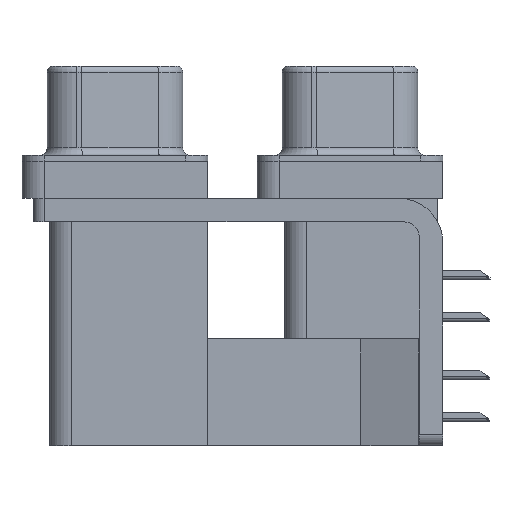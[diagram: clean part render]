
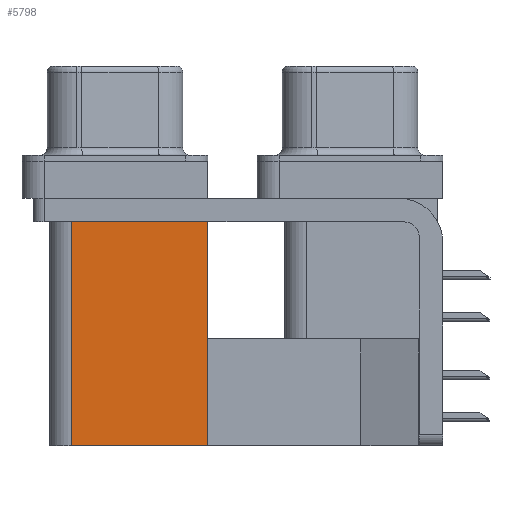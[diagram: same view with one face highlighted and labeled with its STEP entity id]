
A CAD part, left-side view. The second image highlights one B-rep face of the part: STEP entity #5798.
In plain terms, the highlighted planar face has unit normal (-1, 0, 0).
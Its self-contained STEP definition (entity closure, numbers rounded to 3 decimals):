
#100 = DIRECTION ( 'NONE',  ( 1., 0., 0. ) ) ;
#609 = VECTOR ( 'NONE', #3023, 1000. ) ;
#957 = VERTEX_POINT ( 'NONE', #12026 ) ;
#1758 = CARTESIAN_POINT ( 'NONE',  ( 3.79, 9.6, -2.5 ) ) ;
#2810 = LINE ( 'NONE', #4810, #11062 ) ;
#3023 = DIRECTION ( 'NONE',  ( 0., 0., 1. ) ) ;
#3267 = ORIENTED_EDGE ( 'NONE', *, *, #11041, .F. ) ;
#4810 = CARTESIAN_POINT ( 'NONE',  ( 3.79, 18.8, -19.2 ) ) ;
#5171 = DIRECTION ( 'NONE',  ( 0., 1., 0. ) ) ;
#5392 = FACE_OUTER_BOUND ( 'NONE', #19019, .T. ) ;
#5403 = LINE ( 'NONE', #1758, #5768 ) ;
#5515 = DIRECTION ( 'NONE',  ( 0., 0., -1. ) ) ;
#5654 = LINE ( 'NONE', #12859, #22327 ) ;
#5768 = VECTOR ( 'NONE', #19785, 1000. ) ;
#5798 = ADVANCED_FACE ( 'NONE', ( #5392 ), #18022, .F. ) ;
#6360 = DIRECTION ( 'NONE',  ( 0., 0., 1. ) ) ;
#6564 = LINE ( 'NONE', #19173, #609 ) ;
#9059 = CARTESIAN_POINT ( 'NONE',  ( 3.79, 9.6, -19.2 ) ) ;
#9323 = CARTESIAN_POINT ( 'NONE',  ( 3.79, 18.8, -2.5 ) ) ;
#10984 = EDGE_CURVE ( 'NONE', #14609, #16206, #5403, .T. ) ;
#11041 = EDGE_CURVE ( 'NONE', #21202, #957, #5654, .T. ) ;
#11062 = VECTOR ( 'NONE', #6360, 1000. ) ;
#12026 = CARTESIAN_POINT ( 'NONE',  ( 3.79, 18.8, -19.2 ) ) ;
#12859 = CARTESIAN_POINT ( 'NONE',  ( 3.79, 9.6, -19.2 ) ) ;
#13532 = EDGE_CURVE ( 'NONE', #957, #16206, #2810, .T. ) ;
#14609 = VERTEX_POINT ( 'NONE', #16416 ) ;
#15211 = EDGE_CURVE ( 'NONE', #21202, #14609, #6564, .T. ) ;
#16206 = VERTEX_POINT ( 'NONE', #9323 ) ;
#16416 = CARTESIAN_POINT ( 'NONE',  ( 3.79, 9.6, -2.5 ) ) ;
#18022 = PLANE ( 'NONE',  #21932 ) ;
#19019 = EDGE_LOOP ( 'NONE', ( #19382, #21418, #3267, #20746 ) ) ;
#19173 = CARTESIAN_POINT ( 'NONE',  ( 3.79, 9.6, -19.2 ) ) ;
#19382 = ORIENTED_EDGE ( 'NONE', *, *, #10984, .T. ) ;
#19618 = CARTESIAN_POINT ( 'NONE',  ( 3.79, 9.6, -19.2 ) ) ;
#19785 = DIRECTION ( 'NONE',  ( 0., 1., 0. ) ) ;
#20746 = ORIENTED_EDGE ( 'NONE', *, *, #15211, .T. ) ;
#21202 = VERTEX_POINT ( 'NONE', #19618 ) ;
#21418 = ORIENTED_EDGE ( 'NONE', *, *, #13532, .F. ) ;
#21932 = AXIS2_PLACEMENT_3D ( 'NONE', #9059, #100, #5515 ) ;
#22327 = VECTOR ( 'NONE', #5171, 1000. ) ;
